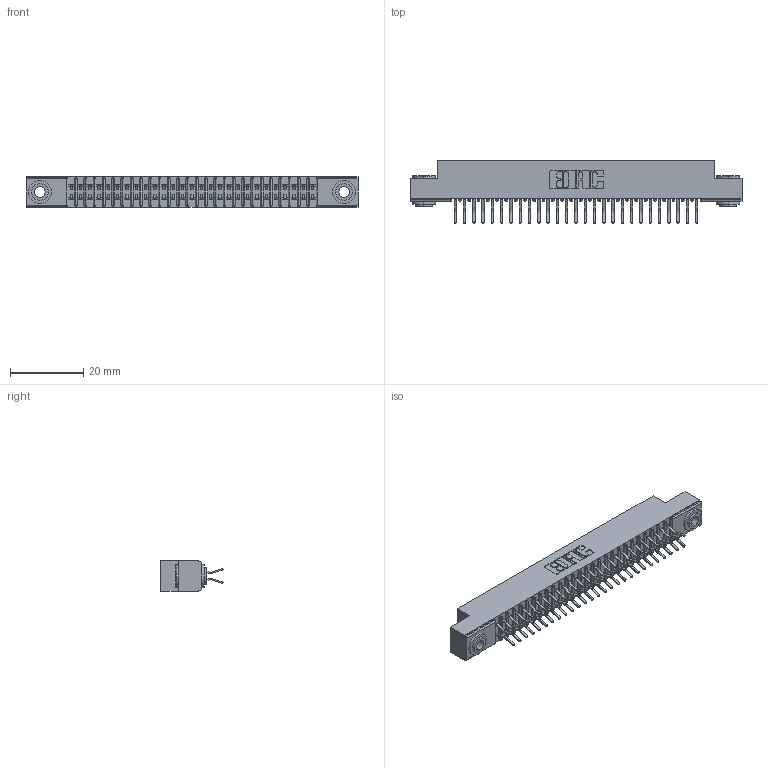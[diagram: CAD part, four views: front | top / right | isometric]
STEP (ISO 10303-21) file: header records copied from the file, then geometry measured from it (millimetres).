
FILE_DESCRIPTION (( 'STEP AP203' ), '1' );
FILE_NAME ('341-054-556-203.STEP', '2018-08-07T14:30:30', ( '' ), ( '' ), 'SwSTEP 2.0', 'SolidWorks 2016', '' );
FILE_SCHEMA (( 'CONFIG_CONTROL_DESIGN' ));
Length unit declared in the file: inch
Products named in the file (4): 341 Part_.156 (3.96) Dia Mounting Holes; 341-292-001_341-292-156; 345-250-002_345-250-002-102; 341-054-556-203
Assembly tree (57 placements, depth 2):
  341-054-556-203
    341 Part_.156 (3.96) Dia Mounting Holes
    341-292-001_341-292-156  x54
    345-250-002_345-250-002-102  x2
Bounding box: 90.81 x 17.07 x 8.38 mm (x, y, z)
Volume: 5174.5 mm3; surface area: 11452.7 mm2
Topology: 57 solids, 57 shells, 3948 faces, 11417 edges, 7406 vertices
Faces by surface type: plane 2252, cylinder 1580, sphere 56, torus 52, cone 8
Entity records: 35879 total; most frequent: CARTESIAN_POINT 5946, ORIENTED_EDGE 5898, DIRECTION 5801, EDGE_CURVE 2949, LINE 2351, VECTOR 2351, VERTEX_POINT 1870, AXIS2_PLACEMENT_3D 1725
